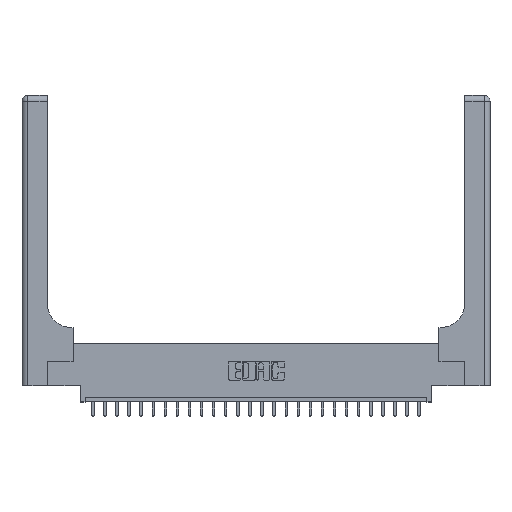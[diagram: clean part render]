
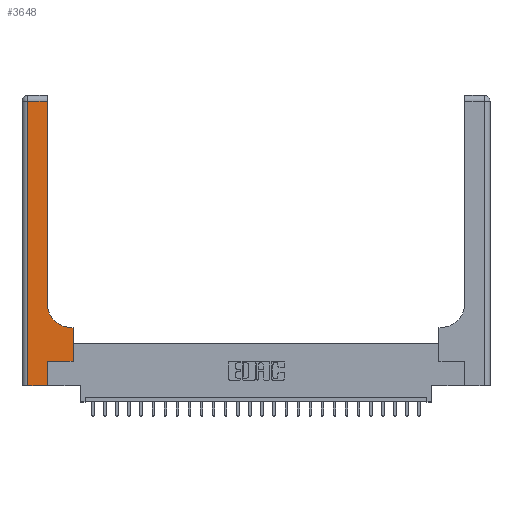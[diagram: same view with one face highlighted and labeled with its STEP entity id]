
A CAD part, top view. The second image highlights one B-rep face of the part: STEP entity #3648.
In plain terms, the highlighted planar face has unit normal (0, 0, 1).
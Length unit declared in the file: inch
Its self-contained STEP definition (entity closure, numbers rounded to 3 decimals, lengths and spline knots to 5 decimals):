
#608 = AXIS2_PLACEMENT_3D ( 'NONE', #13506, #4109, #11859 ) ;
#902 = CARTESIAN_POINT ( 'NONE',  ( 0.528, 0.25, 0.37 ) ) ;
#1398 = AXIS2_PLACEMENT_3D ( 'NONE', #8499, #8377, #6707 ) ;
#1933 = DIRECTION ( 'NONE',  ( -1., 0., 0. ) ) ;
#2191 = LINE ( 'NONE', #12070, #5080 ) ;
#2435 = CARTESIAN_POINT ( 'NONE',  ( 0.26, 0.6, 0.37 ) ) ;
#2494 = ORIENTED_EDGE ( 'NONE', *, *, #23749, .T. ) ;
#2710 = EDGE_CURVE ( 'NONE', #22018, #14963, #19192, .T. ) ;
#2833 = LINE ( 'NONE', #10556, #8062 ) ;
#2986 = CARTESIAN_POINT ( 'NONE',  ( 0.26, 3., 0.37 ) ) ;
#3108 = LINE ( 'NONE', #2986, #7402 ) ;
#3285 = DIRECTION ( 'NONE',  ( 0., 1., 0. ) ) ;
#3531 = DIRECTION ( 'NONE',  ( 1., 0., 0. ) ) ;
#3648 = ADVANCED_FACE ( 'NONE', ( #15856 ), #18240, .F. ) ;
#4079 = DIRECTION ( 'NONE',  ( 0., 1., 0. ) ) ;
#4109 = DIRECTION ( 'NONE',  ( 0., 0., -1. ) ) ;
#5080 = VECTOR ( 'NONE', #4079, 39.37008 ) ;
#5617 = CARTESIAN_POINT ( 'NONE',  ( 0.51, 0.6, 0.37 ) ) ;
#5799 = EDGE_CURVE ( 'NONE', #17429, #5916, #20779, .T. ) ;
#5837 = CARTESIAN_POINT ( 'NONE',  ( 0.06, 3., 0.37 ) ) ;
#5916 = VERTEX_POINT ( 'NONE', #6204 ) ;
#6131 = EDGE_CURVE ( 'NONE', #21219, #24589, #18985, .T. ) ;
#6204 = CARTESIAN_POINT ( 'NONE',  ( 0.528, 0.25, 0.37 ) ) ;
#6707 = DIRECTION ( 'NONE',  ( -1., 0., 0. ) ) ;
#7402 = VECTOR ( 'NONE', #8930, 39.37008 ) ;
#7500 = CARTESIAN_POINT ( 'NONE',  ( 0.26, 0.85, 0.37 ) ) ;
#7998 = CARTESIAN_POINT ( 'NONE',  ( 0.06, 0., 0.37 ) ) ;
#8029 = LINE ( 'NONE', #5837, #13989 ) ;
#8062 = VECTOR ( 'NONE', #1933, 39.37008 ) ;
#8270 = VECTOR ( 'NONE', #12834, 39.37008 ) ;
#8337 = VECTOR ( 'NONE', #10151, 39.37008 ) ;
#8377 = DIRECTION ( 'NONE',  ( 0., 0., -1. ) ) ;
#8499 = CARTESIAN_POINT ( 'NONE',  ( 0., 3., 0.37 ) ) ;
#8758 = CARTESIAN_POINT ( 'NONE',  ( 0.265, 0.25, 0.37 ) ) ;
#8930 = DIRECTION ( 'NONE',  ( 0., 1., 0. ) ) ;
#9059 = EDGE_LOOP ( 'NONE', ( #13308, #13423, #10074, #24370, #2494, #9866, #23447, #24555, #14279 ) ) ;
#9551 = VERTEX_POINT ( 'NONE', #17769 ) ;
#9866 = ORIENTED_EDGE ( 'NONE', *, *, #5799, .T. ) ;
#10074 = ORIENTED_EDGE ( 'NONE', *, *, #25020, .T. ) ;
#10151 = DIRECTION ( 'NONE',  ( -1., 0., 0. ) ) ;
#10556 = CARTESIAN_POINT ( 'NONE',  ( 0., 2.94, 0.37 ) ) ;
#11324 = VECTOR ( 'NONE', #3285, 39.37008 ) ;
#11859 = DIRECTION ( 'NONE',  ( 1., 0., 0. ) ) ;
#12070 = CARTESIAN_POINT ( 'NONE',  ( 0.265, 0., 0.37 ) ) ;
#12834 = DIRECTION ( 'NONE',  ( 1., 0., 0. ) ) ;
#13308 = ORIENTED_EDGE ( 'NONE', *, *, #18190, .T. ) ;
#13423 = ORIENTED_EDGE ( 'NONE', *, *, #14823, .T. ) ;
#13506 = CARTESIAN_POINT ( 'NONE',  ( 0.51, 0.85, 0.37 ) ) ;
#13574 = VERTEX_POINT ( 'NONE', #16741 ) ;
#13861 = DIRECTION ( 'NONE',  ( 0., -1., 0. ) ) ;
#13889 = CARTESIAN_POINT ( 'NONE',  ( 0.265, 0., 0.37 ) ) ;
#13989 = VECTOR ( 'NONE', #13861, 39.37008 ) ;
#14279 = ORIENTED_EDGE ( 'NONE', *, *, #2710, .T. ) ;
#14823 = EDGE_CURVE ( 'NONE', #13574, #9551, #2833, .T. ) ;
#14963 = VERTEX_POINT ( 'NONE', #7500 ) ;
#15067 = CARTESIAN_POINT ( 'NONE',  ( 0.528, 0.6, 0.37 ) ) ;
#15856 = FACE_OUTER_BOUND ( 'NONE', #9059, .T. ) ;
#16246 = EDGE_CURVE ( 'NONE', #5916, #17909, #20635, .T. ) ;
#16706 = VECTOR ( 'NONE', #3531, 39.37008 ) ;
#16722 = CARTESIAN_POINT ( 'NONE',  ( 0., 0., 0.37 ) ) ;
#16741 = CARTESIAN_POINT ( 'NONE',  ( 0.26, 2.94, 0.37 ) ) ;
#17429 = VERTEX_POINT ( 'NONE', #8758 ) ;
#17769 = CARTESIAN_POINT ( 'NONE',  ( 0.06, 2.94, 0.37 ) ) ;
#17909 = VERTEX_POINT ( 'NONE', #15067 ) ;
#18190 = EDGE_CURVE ( 'NONE', #14963, #13574, #3108, .T. ) ;
#18240 = PLANE ( 'NONE',  #1398 ) ;
#18985 = LINE ( 'NONE', #16722, #16706 ) ;
#19024 = CARTESIAN_POINT ( 'NONE',  ( 0.265, 0.25, 0.37 ) ) ;
#19192 = CIRCLE ( 'NONE', #608, 0.25 ) ;
#19787 = LINE ( 'NONE', #2435, #8337 ) ;
#20635 = LINE ( 'NONE', #902, #11324 ) ;
#20779 = LINE ( 'NONE', #19024, #8270 ) ;
#21219 = VERTEX_POINT ( 'NONE', #7998 ) ;
#22018 = VERTEX_POINT ( 'NONE', #5617 ) ;
#23447 = ORIENTED_EDGE ( 'NONE', *, *, #16246, .T. ) ;
#23749 = EDGE_CURVE ( 'NONE', #24589, #17429, #2191, .T. ) ;
#23766 = EDGE_CURVE ( 'NONE', #17909, #22018, #19787, .T. ) ;
#24370 = ORIENTED_EDGE ( 'NONE', *, *, #6131, .T. ) ;
#24555 = ORIENTED_EDGE ( 'NONE', *, *, #23766, .T. ) ;
#24589 = VERTEX_POINT ( 'NONE', #13889 ) ;
#25020 = EDGE_CURVE ( 'NONE', #9551, #21219, #8029, .T. ) ;
